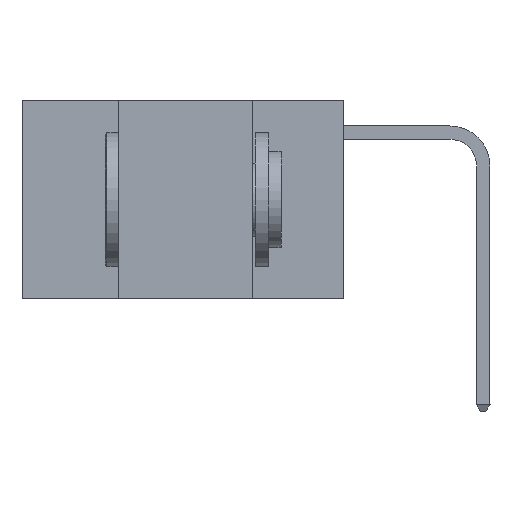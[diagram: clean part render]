
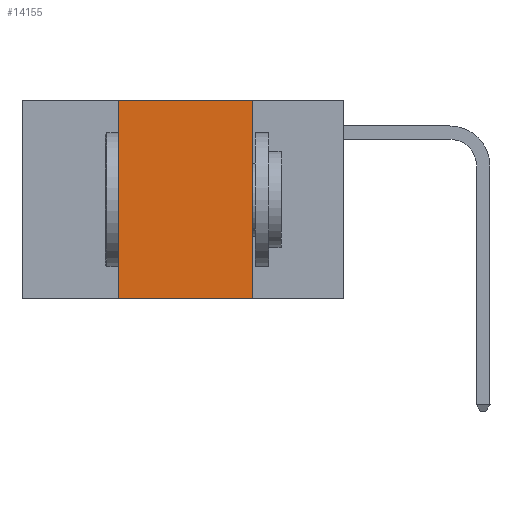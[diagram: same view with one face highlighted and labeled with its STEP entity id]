
A CAD part, left-side view. The second image highlights one B-rep face of the part: STEP entity #14155.
In plain terms, the highlighted planar face has unit normal (-1, 0, 0).
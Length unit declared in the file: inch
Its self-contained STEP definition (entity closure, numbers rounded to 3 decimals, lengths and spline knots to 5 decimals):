
#108 = DIRECTION ( 'NONE',  ( 0., 0., -1. ) ) ;
#339 = ORIENTED_EDGE ( 'NONE', *, *, #7669, .F. ) ;
#465 = ORIENTED_EDGE ( 'NONE', *, *, #3341, .T. ) ;
#780 = LINE ( 'NONE', #9503, #10875 ) ;
#1060 = CARTESIAN_POINT ( 'NONE',  ( 0., 0.6, 0. ) ) ;
#1283 = EDGE_LOOP ( 'NONE', ( #14068, #7402, #339, #465 ) ) ;
#2022 = VECTOR ( 'NONE', #13618, 39.37008 ) ;
#2448 = VERTEX_POINT ( 'NONE', #4631 ) ;
#3137 = VERTEX_POINT ( 'NONE', #5721 ) ;
#3341 = EDGE_CURVE ( 'NONE', #5621, #10012, #3760, .T. ) ;
#3760 = LINE ( 'NONE', #12459, #2022 ) ;
#4430 = PLANE ( 'NONE',  #4945 ) ;
#4631 = CARTESIAN_POINT ( 'NONE',  ( 0., 0.42, 0. ) ) ;
#4945 = AXIS2_PLACEMENT_3D ( 'NONE', #1060, #10965, #108 ) ;
#5177 = DIRECTION ( 'NONE',  ( 0., 0., 1. ) ) ;
#5330 = VECTOR ( 'NONE', #10453, 39.37008 ) ;
#5561 = EDGE_CURVE ( 'NONE', #2448, #3137, #10723, .T. ) ;
#5621 = VERTEX_POINT ( 'NONE', #9653 ) ;
#5721 = CARTESIAN_POINT ( 'NONE',  ( 0., 0.17, 0. ) ) ;
#5832 = LINE ( 'NONE', #10443, #13185 ) ;
#7059 = DIRECTION ( 'NONE',  ( 0., 0., -1. ) ) ;
#7402 = ORIENTED_EDGE ( 'NONE', *, *, #5561, .F. ) ;
#7669 = EDGE_CURVE ( 'NONE', #5621, #2448, #780, .T. ) ;
#9503 = CARTESIAN_POINT ( 'NONE',  ( 0., 0.42, 0. ) ) ;
#9653 = CARTESIAN_POINT ( 'NONE',  ( 0., 0.42, -0.37 ) ) ;
#10012 = VERTEX_POINT ( 'NONE', #11811 ) ;
#10443 = CARTESIAN_POINT ( 'NONE',  ( 0., 0.17, 0. ) ) ;
#10453 = DIRECTION ( 'NONE',  ( 0., -1., 0. ) ) ;
#10723 = LINE ( 'NONE', #11502, #5330 ) ;
#10875 = VECTOR ( 'NONE', #5177, 39.37008 ) ;
#10965 = DIRECTION ( 'NONE',  ( 1., 0., 0. ) ) ;
#11502 = CARTESIAN_POINT ( 'NONE',  ( 0., 0.6, 0. ) ) ;
#11811 = CARTESIAN_POINT ( 'NONE',  ( 0., 0.17, -0.37 ) ) ;
#11972 = FACE_OUTER_BOUND ( 'NONE', #1283, .T. ) ;
#12459 = CARTESIAN_POINT ( 'NONE',  ( 0., 0.6, -0.37 ) ) ;
#13185 = VECTOR ( 'NONE', #7059, 39.37008 ) ;
#13379 = EDGE_CURVE ( 'NONE', #3137, #10012, #5832, .T. ) ;
#13618 = DIRECTION ( 'NONE',  ( 0., -1., 0. ) ) ;
#14068 = ORIENTED_EDGE ( 'NONE', *, *, #13379, .F. ) ;
#14155 = ADVANCED_FACE ( 'NONE', ( #11972 ), #4430, .F. ) ;
